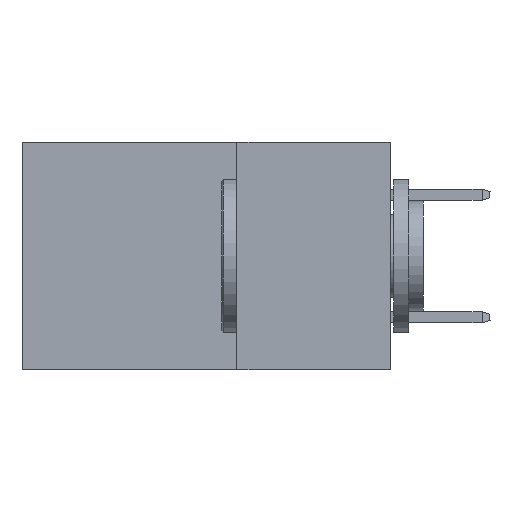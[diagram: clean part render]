
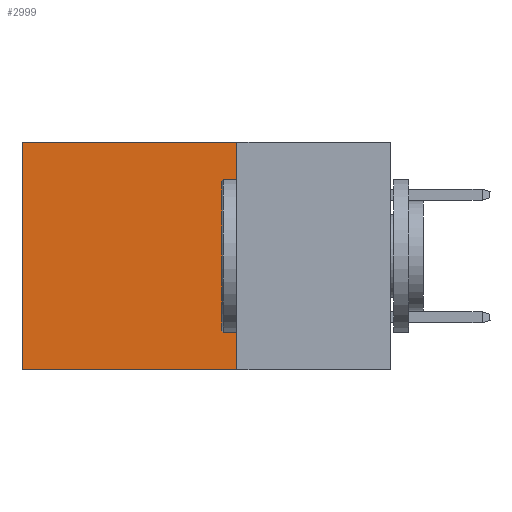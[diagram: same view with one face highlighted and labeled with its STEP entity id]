
A CAD part, left-side view. The second image highlights one B-rep face of the part: STEP entity #2999.
In plain terms, the highlighted planar face has unit normal (-1, 0, 0).
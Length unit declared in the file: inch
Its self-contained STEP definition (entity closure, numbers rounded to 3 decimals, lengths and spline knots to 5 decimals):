
#288 = LINE ( 'NONE', #8882, #7099 ) ;
#345 = EDGE_CURVE ( 'NONE', #4409, #7883, #6704, .T. ) ;
#389 = VECTOR ( 'NONE', #8371, 39.37008 ) ;
#392 = VECTOR ( 'NONE', #6281, 39.37008 ) ;
#1680 = FACE_OUTER_BOUND ( 'NONE', #6154, .T. ) ;
#2522 = DIRECTION ( 'NONE',  ( 0., 1., 0. ) ) ;
#2687 = CARTESIAN_POINT ( 'NONE',  ( 0.2875, 0.25, -0.37 ) ) ;
#2999 = ADVANCED_FACE ( 'NONE', ( #1680 ), #3080, .F. ) ;
#3080 = PLANE ( 'NONE',  #4071 ) ;
#3278 = CARTESIAN_POINT ( 'NONE',  ( 0.2875, 0.25, -0.37 ) ) ;
#3577 = ORIENTED_EDGE ( 'NONE', *, *, #345, .F. ) ;
#3644 = ORIENTED_EDGE ( 'NONE', *, *, #8588, .T. ) ;
#4007 = DIRECTION ( 'NONE',  ( 0., 0., -1. ) ) ;
#4071 = AXIS2_PLACEMENT_3D ( 'NONE', #8581, #4373, #4583 ) ;
#4113 = CARTESIAN_POINT ( 'NONE',  ( 0.2875, 0.6, 0. ) ) ;
#4244 = ORIENTED_EDGE ( 'NONE', *, *, #5499, .F. ) ;
#4277 = VERTEX_POINT ( 'NONE', #4113 ) ;
#4373 = DIRECTION ( 'NONE',  ( 1., 0., 0. ) ) ;
#4409 = VERTEX_POINT ( 'NONE', #2687 ) ;
#4583 = DIRECTION ( 'NONE',  ( 0., 0., -1. ) ) ;
#5030 = EDGE_CURVE ( 'NONE', #4277, #7883, #288, .T. ) ;
#5499 = EDGE_CURVE ( 'NONE', #7373, #4409, #6959, .T. ) ;
#6154 = EDGE_LOOP ( 'NONE', ( #9925, #3577, #4244, #3644 ) ) ;
#6281 = DIRECTION ( 'NONE',  ( 0., 0., -1. ) ) ;
#6704 = LINE ( 'NONE', #3278, #8605 ) ;
#6959 = LINE ( 'NONE', #7049, #392 ) ;
#7049 = CARTESIAN_POINT ( 'NONE',  ( 0.2875, 0.25, 0. ) ) ;
#7099 = VECTOR ( 'NONE', #4007, 39.37008 ) ;
#7373 = VERTEX_POINT ( 'NONE', #10302 ) ;
#7603 = CARTESIAN_POINT ( 'NONE',  ( 0.2875, 0.25, 0. ) ) ;
#7883 = VERTEX_POINT ( 'NONE', #9845 ) ;
#8371 = DIRECTION ( 'NONE',  ( 0., 1., 0. ) ) ;
#8581 = CARTESIAN_POINT ( 'NONE',  ( 0.2875, 0.25, 0. ) ) ;
#8588 = EDGE_CURVE ( 'NONE', #7373, #4277, #8985, .T. ) ;
#8605 = VECTOR ( 'NONE', #2522, 39.37008 ) ;
#8882 = CARTESIAN_POINT ( 'NONE',  ( 0.2875, 0.6, 0. ) ) ;
#8985 = LINE ( 'NONE', #7603, #389 ) ;
#9845 = CARTESIAN_POINT ( 'NONE',  ( 0.2875, 0.6, -0.37 ) ) ;
#9925 = ORIENTED_EDGE ( 'NONE', *, *, #5030, .T. ) ;
#10302 = CARTESIAN_POINT ( 'NONE',  ( 0.2875, 0.25, 0. ) ) ;
